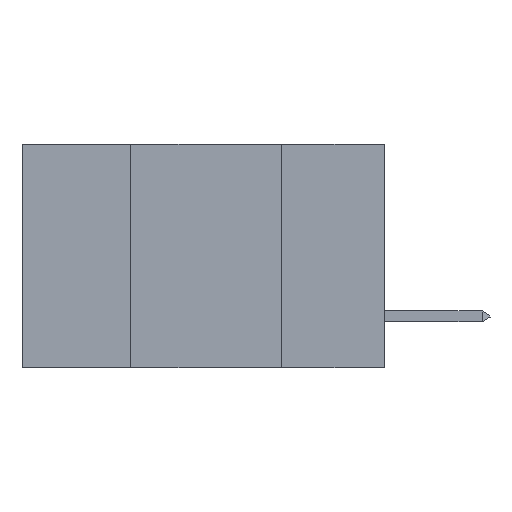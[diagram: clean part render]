
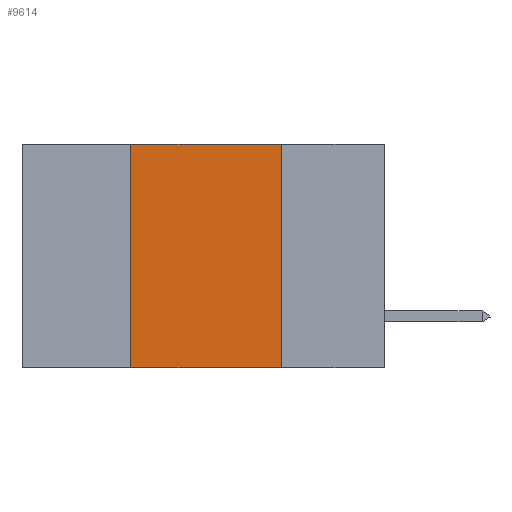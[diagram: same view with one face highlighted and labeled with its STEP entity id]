
A CAD part, left-side view. The second image highlights one B-rep face of the part: STEP entity #9614.
In plain terms, the highlighted planar face has unit normal (-1, 0, 0).
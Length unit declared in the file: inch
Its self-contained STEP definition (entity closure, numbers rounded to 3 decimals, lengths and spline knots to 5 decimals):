
#7 = FACE_OUTER_BOUND ( 'NONE', #9479, .T. ) ;
#348 = VERTEX_POINT ( 'NONE', #1775 ) ;
#634 = CARTESIAN_POINT ( 'NONE',  ( 0., 0.17, -0.37 ) ) ;
#900 = DIRECTION ( 'NONE',  ( 1., 0., 0. ) ) ;
#1646 = CARTESIAN_POINT ( 'NONE',  ( 0., 0.6, -0.37 ) ) ;
#1775 = CARTESIAN_POINT ( 'NONE',  ( 0., 0.42, -0.37 ) ) ;
#2244 = ORIENTED_EDGE ( 'NONE', *, *, #13650, .T. ) ;
#2566 = VERTEX_POINT ( 'NONE', #634 ) ;
#3236 = PLANE ( 'NONE',  #4447 ) ;
#3371 = DIRECTION ( 'NONE',  ( 0., -1., 0. ) ) ;
#4447 = AXIS2_PLACEMENT_3D ( 'NONE', #5366, #900, #17827 ) ;
#4628 = CARTESIAN_POINT ( 'NONE',  ( 0., 0.17, 0. ) ) ;
#5366 = CARTESIAN_POINT ( 'NONE',  ( 0., 0.6, 0. ) ) ;
#6495 = ORIENTED_EDGE ( 'NONE', *, *, #23736, .F. ) ;
#6968 = EDGE_CURVE ( 'NONE', #21757, #16037, #20400, .T. ) ;
#7051 = VECTOR ( 'NONE', #26901, 39.37008 ) ;
#7160 = ORIENTED_EDGE ( 'NONE', *, *, #11772, .F. ) ;
#7779 = LINE ( 'NONE', #4628, #12786 ) ;
#8043 = LINE ( 'NONE', #18420, #7051 ) ;
#9479 = EDGE_LOOP ( 'NONE', ( #6495, #26102, #7160, #2244 ) ) ;
#9614 = ADVANCED_FACE ( 'NONE', ( #7 ), #3236, .F. ) ;
#11770 = CARTESIAN_POINT ( 'NONE',  ( 0., 0.42, 0. ) ) ;
#11772 = EDGE_CURVE ( 'NONE', #348, #21757, #8043, .T. ) ;
#12786 = VECTOR ( 'NONE', #21804, 39.37008 ) ;
#12993 = VECTOR ( 'NONE', #22737, 39.37008 ) ;
#13650 = EDGE_CURVE ( 'NONE', #348, #2566, #20615, .T. ) ;
#14800 = VECTOR ( 'NONE', #3371, 39.37008 ) ;
#16037 = VERTEX_POINT ( 'NONE', #22755 ) ;
#17827 = DIRECTION ( 'NONE',  ( 0., 0., -1. ) ) ;
#18420 = CARTESIAN_POINT ( 'NONE',  ( 0., 0.42, 0. ) ) ;
#20400 = LINE ( 'NONE', #21769, #14800 ) ;
#20615 = LINE ( 'NONE', #1646, #12993 ) ;
#21757 = VERTEX_POINT ( 'NONE', #11770 ) ;
#21769 = CARTESIAN_POINT ( 'NONE',  ( 0., 0.6, 0. ) ) ;
#21804 = DIRECTION ( 'NONE',  ( 0., 0., -1. ) ) ;
#22737 = DIRECTION ( 'NONE',  ( 0., -1., 0. ) ) ;
#22755 = CARTESIAN_POINT ( 'NONE',  ( 0., 0.17, 0. ) ) ;
#23736 = EDGE_CURVE ( 'NONE', #16037, #2566, #7779, .T. ) ;
#26102 = ORIENTED_EDGE ( 'NONE', *, *, #6968, .F. ) ;
#26901 = DIRECTION ( 'NONE',  ( 0., 0., 1. ) ) ;
